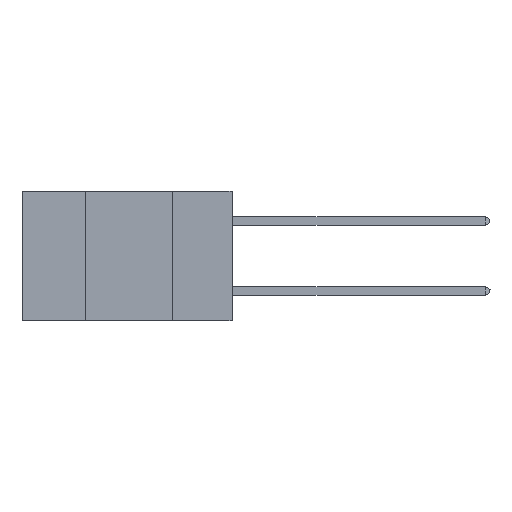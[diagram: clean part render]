
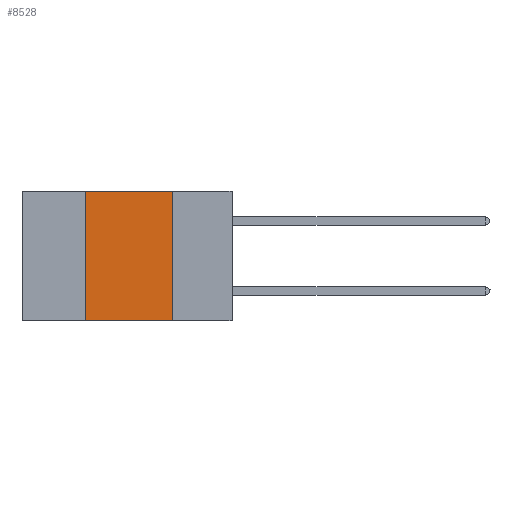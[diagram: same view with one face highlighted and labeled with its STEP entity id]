
A CAD part, left-side view. The second image highlights one B-rep face of the part: STEP entity #8528.
In plain terms, the highlighted planar face has unit normal (-1, 0, 0).
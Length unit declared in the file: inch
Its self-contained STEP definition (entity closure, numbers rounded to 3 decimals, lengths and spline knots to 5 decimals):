
#947 = VECTOR ( 'NONE', #42468, 39.37008 ) ;
#2486 = CARTESIAN_POINT ( 'NONE',  ( 0., 0.6, 0. ) ) ;
#3226 = VECTOR ( 'NONE', #36547, 39.37008 ) ;
#3813 = CARTESIAN_POINT ( 'NONE',  ( 0., 0.42, 0. ) ) ;
#4562 = VECTOR ( 'NONE', #9530, 39.37008 ) ;
#8528 = ADVANCED_FACE ( 'NONE', ( #24723 ), #8828, .F. ) ;
#8828 = PLANE ( 'NONE',  #29835 ) ;
#9256 = DIRECTION ( 'NONE',  ( 1., 0., 0. ) ) ;
#9530 = DIRECTION ( 'NONE',  ( 0., 0., -1. ) ) ;
#10762 = VERTEX_POINT ( 'NONE', #31097 ) ;
#10883 = LINE ( 'NONE', #29172, #41890 ) ;
#11149 = CARTESIAN_POINT ( 'NONE',  ( 0., 0.17, -0.37 ) ) ;
#14001 = EDGE_CURVE ( 'NONE', #18597, #25212, #10883, .T. ) ;
#15338 = ORIENTED_EDGE ( 'NONE', *, *, #14001, .F. ) ;
#16799 = CARTESIAN_POINT ( 'NONE',  ( 0., 0.6, -0.37 ) ) ;
#18597 = VERTEX_POINT ( 'NONE', #36416 ) ;
#21198 = EDGE_CURVE ( 'NONE', #10762, #21739, #29325, .T. ) ;
#21739 = VERTEX_POINT ( 'NONE', #11149 ) ;
#22005 = ORIENTED_EDGE ( 'NONE', *, *, #21198, .F. ) ;
#23661 = ORIENTED_EDGE ( 'NONE', *, *, #36942, .F. ) ;
#24723 = FACE_OUTER_BOUND ( 'NONE', #40913, .T. ) ;
#25212 = VERTEX_POINT ( 'NONE', #3813 ) ;
#25878 = DIRECTION ( 'NONE',  ( 0., 0., 1. ) ) ;
#29172 = CARTESIAN_POINT ( 'NONE',  ( 0., 0.42, 0. ) ) ;
#29267 = EDGE_CURVE ( 'NONE', #18597, #21739, #34758, .T. ) ;
#29272 = CARTESIAN_POINT ( 'NONE',  ( 0., 0.17, 0. ) ) ;
#29325 = LINE ( 'NONE', #29272, #4562 ) ;
#29835 = AXIS2_PLACEMENT_3D ( 'NONE', #31902, #9256, #38738 ) ;
#31097 = CARTESIAN_POINT ( 'NONE',  ( 0., 0.17, 0. ) ) ;
#31902 = CARTESIAN_POINT ( 'NONE',  ( 0., 0.6, 0. ) ) ;
#33065 = ORIENTED_EDGE ( 'NONE', *, *, #29267, .T. ) ;
#34758 = LINE ( 'NONE', #16799, #3226 ) ;
#35565 = LINE ( 'NONE', #2486, #947 ) ;
#36416 = CARTESIAN_POINT ( 'NONE',  ( 0., 0.42, -0.37 ) ) ;
#36547 = DIRECTION ( 'NONE',  ( 0., -1., 0. ) ) ;
#36942 = EDGE_CURVE ( 'NONE', #25212, #10762, #35565, .T. ) ;
#38738 = DIRECTION ( 'NONE',  ( 0., 0., -1. ) ) ;
#40913 = EDGE_LOOP ( 'NONE', ( #22005, #23661, #15338, #33065 ) ) ;
#41890 = VECTOR ( 'NONE', #25878, 39.37008 ) ;
#42468 = DIRECTION ( 'NONE',  ( 0., -1., 0. ) ) ;
